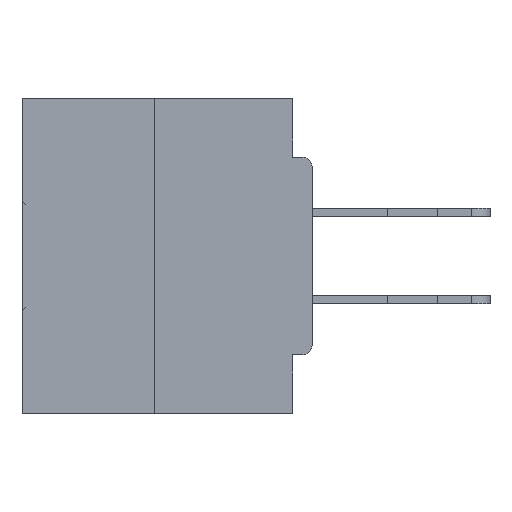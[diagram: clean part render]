
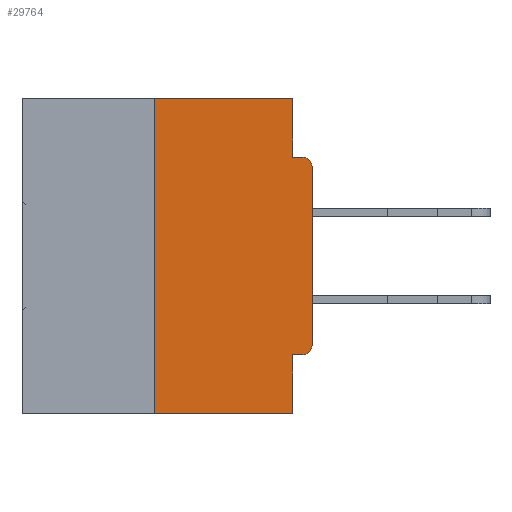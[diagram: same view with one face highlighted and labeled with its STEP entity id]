
A CAD part, left-side view. The second image highlights one B-rep face of the part: STEP entity #29764.
In plain terms, the highlighted planar face has unit normal (-1, 0, 0).
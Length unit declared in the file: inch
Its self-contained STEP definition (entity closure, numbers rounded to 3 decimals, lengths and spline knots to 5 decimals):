
#472 = CARTESIAN_POINT ( 'NONE',  ( 0., 0., 0. ) ) ;
#682 = DIRECTION ( 'NONE',  ( 0., 0., -1. ) ) ;
#897 = DIRECTION ( 'NONE',  ( 0., 0., 1. ) ) ;
#916 = VERTEX_POINT ( 'NONE', #25498 ) ;
#1063 = EDGE_CURVE ( 'NONE', #34072, #25461, #23345, .T. ) ;
#1597 = ORIENTED_EDGE ( 'NONE', *, *, #39014, .F. ) ;
#1684 = EDGE_CURVE ( 'NONE', #22144, #25461, #7352, .T. ) ;
#4122 = CARTESIAN_POINT ( 'NONE',  ( 0., 0.015, -0.1085 ) ) ;
#4455 = CARTESIAN_POINT ( 'NONE',  ( 0., 0.46, 0. ) ) ;
#4553 = DIRECTION ( 'NONE',  ( 0., 0., -1. ) ) ;
#5096 = VECTOR ( 'NONE', #34020, 39.37008 ) ;
#5412 = VERTEX_POINT ( 'NONE', #33273 ) ;
#5589 = ORIENTED_EDGE ( 'NONE', *, *, #32617, .T. ) ;
#5764 = CARTESIAN_POINT ( 'NONE',  ( 0., 0., -0.0935 ) ) ;
#5949 = CARTESIAN_POINT ( 'NONE',  ( 0., 0.031, -0.4065 ) ) ;
#6496 = AXIS2_PLACEMENT_3D ( 'NONE', #11510, #38024, #37887 ) ;
#7352 = LINE ( 'NONE', #26853, #16064 ) ;
#7441 = DIRECTION ( 'NONE',  ( -1., 0., 0. ) ) ;
#8365 = DIRECTION ( 'NONE',  ( 0., 0., -1. ) ) ;
#9075 = DIRECTION ( 'NONE',  ( 0., -1., 0. ) ) ;
#9501 = VERTEX_POINT ( 'NONE', #39639 ) ;
#10555 = ORIENTED_EDGE ( 'NONE', *, *, #25409, .F. ) ;
#11510 = CARTESIAN_POINT ( 'NONE',  ( 0., 0.015, -0.3915 ) ) ;
#13206 = FACE_OUTER_BOUND ( 'NONE', #16088, .T. ) ;
#13540 = CARTESIAN_POINT ( 'NONE',  ( 0., 0., -0.3915 ) ) ;
#13989 = CIRCLE ( 'NONE', #6496, 0.015 ) ;
#14112 = LINE ( 'NONE', #34448, #15577 ) ;
#15577 = VECTOR ( 'NONE', #8365, 39.37008 ) ;
#15875 = LINE ( 'NONE', #39776, #5096 ) ;
#16064 = VECTOR ( 'NONE', #30145, 39.37008 ) ;
#16088 = EDGE_LOOP ( 'NONE', ( #17453, #10555, #19069, #20452, #21630, #5589, #34034, #36830, #1597, #28374 ) ) ;
#17408 = PLANE ( 'NONE',  #17498 ) ;
#17453 = ORIENTED_EDGE ( 'NONE', *, *, #41015, .F. ) ;
#17498 = AXIS2_PLACEMENT_3D ( 'NONE', #23842, #36735, #682 ) ;
#18622 = VERTEX_POINT ( 'NONE', #13540 ) ;
#18682 = LINE ( 'NONE', #24828, #30968 ) ;
#19069 = ORIENTED_EDGE ( 'NONE', *, *, #1063, .T. ) ;
#19539 = CARTESIAN_POINT ( 'NONE',  ( 0., 0.25, 0. ) ) ;
#19884 = AXIS2_PLACEMENT_3D ( 'NONE', #4122, #7441, #4553 ) ;
#20452 = ORIENTED_EDGE ( 'NONE', *, *, #1684, .F. ) ;
#20502 = LINE ( 'NONE', #4455, #27676 ) ;
#21630 = ORIENTED_EDGE ( 'NONE', *, *, #34378, .F. ) ;
#21785 = VECTOR ( 'NONE', #897, 39.37008 ) ;
#21829 = DIRECTION ( 'NONE',  ( 0., 0., 1. ) ) ;
#22144 = VERTEX_POINT ( 'NONE', #5949 ) ;
#22203 = LINE ( 'NONE', #5764, #29364 ) ;
#22359 = CARTESIAN_POINT ( 'NONE',  ( 0., 0.46, -0.5 ) ) ;
#22815 = CARTESIAN_POINT ( 'NONE',  ( 0., 0.015, -0.4065 ) ) ;
#23345 = LINE ( 'NONE', #22359, #33050 ) ;
#23842 = CARTESIAN_POINT ( 'NONE',  ( 0., 0.46, 0. ) ) ;
#24274 = DIRECTION ( 'NONE',  ( 0., -1., 0. ) ) ;
#24828 = CARTESIAN_POINT ( 'NONE',  ( 0., 0.25, 0. ) ) ;
#25409 = EDGE_CURVE ( 'NONE', #34072, #40684, #18682, .T. ) ;
#25461 = VERTEX_POINT ( 'NONE', #25528 ) ;
#25498 = CARTESIAN_POINT ( 'NONE',  ( 0., 0., -0.1085 ) ) ;
#25528 = CARTESIAN_POINT ( 'NONE',  ( 0., 0.031, -0.5 ) ) ;
#25921 = DIRECTION ( 'NONE',  ( 0., -1., 0. ) ) ;
#26520 = CIRCLE ( 'NONE', #19884, 0.015 ) ;
#26853 = CARTESIAN_POINT ( 'NONE',  ( 0., 0.031, -0.5 ) ) ;
#26961 = CARTESIAN_POINT ( 'NONE',  ( 0., 0.031, 0. ) ) ;
#27676 = VECTOR ( 'NONE', #24274, 39.37008 ) ;
#27783 = VERTEX_POINT ( 'NONE', #26961 ) ;
#28374 = ORIENTED_EDGE ( 'NONE', *, *, #31389, .F. ) ;
#28892 = CARTESIAN_POINT ( 'NONE',  ( 0., 0.25, -0.5 ) ) ;
#29364 = VECTOR ( 'NONE', #9075, 39.37008 ) ;
#29764 = ADVANCED_FACE ( 'NONE', ( #13206 ), #17408, .F. ) ;
#30145 = DIRECTION ( 'NONE',  ( 0., 0., -1. ) ) ;
#30968 = VECTOR ( 'NONE', #21829, 39.37008 ) ;
#31389 = EDGE_CURVE ( 'NONE', #27783, #9501, #14112, .T. ) ;
#32617 = EDGE_CURVE ( 'NONE', #39540, #18622, #13989, .T. ) ;
#33050 = VECTOR ( 'NONE', #25921, 39.37008 ) ;
#33273 = CARTESIAN_POINT ( 'NONE',  ( 0., 0.015, -0.0935 ) ) ;
#34020 = DIRECTION ( 'NONE',  ( 0., 1., 0. ) ) ;
#34034 = ORIENTED_EDGE ( 'NONE', *, *, #37554, .T. ) ;
#34072 = VERTEX_POINT ( 'NONE', #28892 ) ;
#34378 = EDGE_CURVE ( 'NONE', #39540, #22144, #15875, .T. ) ;
#34448 = CARTESIAN_POINT ( 'NONE',  ( 0., 0.031, 0. ) ) ;
#36020 = EDGE_CURVE ( 'NONE', #916, #5412, #26520, .T. ) ;
#36735 = DIRECTION ( 'NONE',  ( 1., 0., 0. ) ) ;
#36830 = ORIENTED_EDGE ( 'NONE', *, *, #36020, .T. ) ;
#37554 = EDGE_CURVE ( 'NONE', #18622, #916, #37719, .T. ) ;
#37719 = LINE ( 'NONE', #472, #21785 ) ;
#37887 = DIRECTION ( 'NONE',  ( 0., 0., -1. ) ) ;
#38024 = DIRECTION ( 'NONE',  ( -1., 0., 0. ) ) ;
#39014 = EDGE_CURVE ( 'NONE', #9501, #5412, #22203, .T. ) ;
#39540 = VERTEX_POINT ( 'NONE', #22815 ) ;
#39639 = CARTESIAN_POINT ( 'NONE',  ( 0., 0.031, -0.0935 ) ) ;
#39776 = CARTESIAN_POINT ( 'NONE',  ( 0., 0., -0.4065 ) ) ;
#40684 = VERTEX_POINT ( 'NONE', #19539 ) ;
#41015 = EDGE_CURVE ( 'NONE', #40684, #27783, #20502, .T. ) ;
